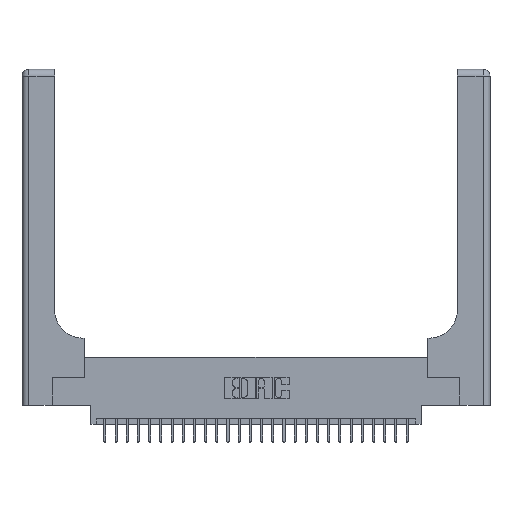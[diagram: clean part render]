
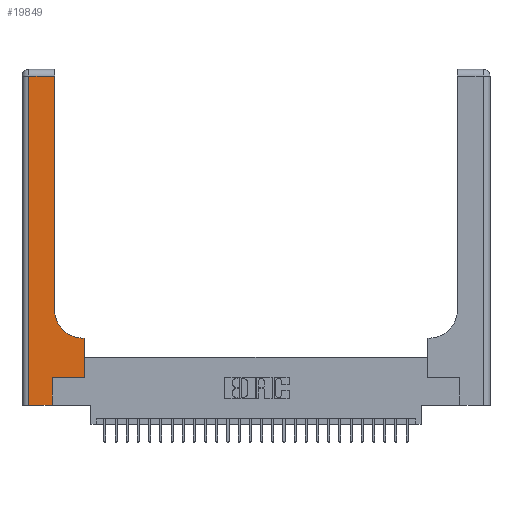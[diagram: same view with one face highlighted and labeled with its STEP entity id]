
A CAD part, top view. The second image highlights one B-rep face of the part: STEP entity #19849.
In plain terms, the highlighted planar face has unit normal (0, 0, 1).
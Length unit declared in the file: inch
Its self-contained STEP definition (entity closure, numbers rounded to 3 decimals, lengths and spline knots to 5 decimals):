
#695 = ORIENTED_EDGE ( 'NONE', *, *, #17279, .T. ) ;
#705 = CARTESIAN_POINT ( 'NONE',  ( 0.269, 0., 0.37 ) ) ;
#976 = VERTEX_POINT ( 'NONE', #12389 ) ;
#1508 = VERTEX_POINT ( 'NONE', #21222 ) ;
#1561 = CARTESIAN_POINT ( 'NONE',  ( 0.269, 0.25, 0.37 ) ) ;
#1582 = CARTESIAN_POINT ( 'NONE',  ( 0.06, 2.94, 0.37 ) ) ;
#2158 = CARTESIAN_POINT ( 'NONE',  ( 0.06, 3., 0.37 ) ) ;
#2803 = FACE_OUTER_BOUND ( 'NONE', #26682, .T. ) ;
#2903 = VERTEX_POINT ( 'NONE', #705 ) ;
#3020 = DIRECTION ( 'NONE',  ( 0., 1., 0. ) ) ;
#3133 = CARTESIAN_POINT ( 'NONE',  ( 0.5415, 0.85, 0.37 ) ) ;
#3199 = LINE ( 'NONE', #19213, #16576 ) ;
#3409 = VECTOR ( 'NONE', #8537, 39.37008 ) ;
#3973 = CARTESIAN_POINT ( 'NONE',  ( 0.2915, 0.85, 0.37 ) ) ;
#4319 = EDGE_CURVE ( 'NONE', #24713, #976, #20401, .T. ) ;
#5251 = VECTOR ( 'NONE', #23430, 39.37008 ) ;
#5928 = ORIENTED_EDGE ( 'NONE', *, *, #14879, .T. ) ;
#6077 = EDGE_CURVE ( 'NONE', #976, #27820, #9397, .T. ) ;
#6463 = CARTESIAN_POINT ( 'NONE',  ( 0., 2.94, 0.37 ) ) ;
#7162 = LINE ( 'NONE', #2158, #20213 ) ;
#7233 = VERTEX_POINT ( 'NONE', #18867 ) ;
#7284 = EDGE_CURVE ( 'NONE', #23984, #1508, #7162, .T. ) ;
#7417 = ORIENTED_EDGE ( 'NONE', *, *, #4319, .T. ) ;
#7922 = EDGE_CURVE ( 'NONE', #27820, #7233, #22665, .T. ) ;
#8462 = AXIS2_PLACEMENT_3D ( 'NONE', #21516, #21420, #23816 ) ;
#8537 = DIRECTION ( 'NONE',  ( -1., 0., 0. ) ) ;
#8786 = DIRECTION ( 'NONE',  ( 0., -1., 0. ) ) ;
#9397 = LINE ( 'NONE', #21067, #14976 ) ;
#9535 = DIRECTION ( 'NONE',  ( 0., 1., 0. ) ) ;
#9576 = EDGE_CURVE ( 'NONE', #7233, #25242, #14083, .T. ) ;
#10466 = LINE ( 'NONE', #11549, #18860 ) ;
#10590 = ORIENTED_EDGE ( 'NONE', *, *, #9576, .T. ) ;
#10990 = VECTOR ( 'NONE', #9535, 39.37008 ) ;
#11549 = CARTESIAN_POINT ( 'NONE',  ( 0., 0., 0.37 ) ) ;
#12389 = CARTESIAN_POINT ( 'NONE',  ( 0.5585, 0.25, 0.37 ) ) ;
#13923 = LINE ( 'NONE', #6463, #3409 ) ;
#14083 = CIRCLE ( 'NONE', #21953, 0.25 ) ;
#14301 = EDGE_CURVE ( 'NONE', #24457, #23984, #13923, .T. ) ;
#14713 = CARTESIAN_POINT ( 'NONE',  ( 0.2915, 3., 0.37 ) ) ;
#14879 = EDGE_CURVE ( 'NONE', #1508, #2903, #10466, .T. ) ;
#14976 = VECTOR ( 'NONE', #3020, 39.37008 ) ;
#15529 = CARTESIAN_POINT ( 'NONE',  ( 0.5585, 0.6, 0.37 ) ) ;
#16576 = VECTOR ( 'NONE', #24003, 39.37008 ) ;
#17279 = EDGE_CURVE ( 'NONE', #25242, #24457, #27245, .T. ) ;
#18101 = VECTOR ( 'NONE', #26545, 39.37008 ) ;
#18860 = VECTOR ( 'NONE', #28061, 39.37008 ) ;
#18867 = CARTESIAN_POINT ( 'NONE',  ( 0.5415, 0.6, 0.37 ) ) ;
#19060 = ORIENTED_EDGE ( 'NONE', *, *, #7922, .T. ) ;
#19213 = CARTESIAN_POINT ( 'NONE',  ( 0.269, 0., 0.37 ) ) ;
#19849 = ADVANCED_FACE ( 'NONE', ( #2803 ), #28256, .F. ) ;
#20213 = VECTOR ( 'NONE', #8786, 39.37008 ) ;
#20401 = LINE ( 'NONE', #21445, #5251 ) ;
#20995 = DIRECTION ( 'NONE',  ( 0., 0., -1. ) ) ;
#21067 = CARTESIAN_POINT ( 'NONE',  ( 0.5585, 0.25, 0.37 ) ) ;
#21222 = CARTESIAN_POINT ( 'NONE',  ( 0.06, 0., 0.37 ) ) ;
#21420 = DIRECTION ( 'NONE',  ( 0., 0., -1. ) ) ;
#21430 = ORIENTED_EDGE ( 'NONE', *, *, #25839, .T. ) ;
#21445 = CARTESIAN_POINT ( 'NONE',  ( 0.269, 0.25, 0.37 ) ) ;
#21516 = CARTESIAN_POINT ( 'NONE',  ( 0., 3., 0.37 ) ) ;
#21953 = AXIS2_PLACEMENT_3D ( 'NONE', #3133, #20995, #25650 ) ;
#21979 = ORIENTED_EDGE ( 'NONE', *, *, #6077, .T. ) ;
#22665 = LINE ( 'NONE', #24667, #18101 ) ;
#23430 = DIRECTION ( 'NONE',  ( 1., 0., 0. ) ) ;
#23816 = DIRECTION ( 'NONE',  ( -1., 0., 0. ) ) ;
#23984 = VERTEX_POINT ( 'NONE', #1582 ) ;
#24003 = DIRECTION ( 'NONE',  ( 0., 1., 0. ) ) ;
#24457 = VERTEX_POINT ( 'NONE', #28130 ) ;
#24667 = CARTESIAN_POINT ( 'NONE',  ( 0.2915, 0.6, 0.37 ) ) ;
#24713 = VERTEX_POINT ( 'NONE', #1561 ) ;
#24883 = ORIENTED_EDGE ( 'NONE', *, *, #14301, .T. ) ;
#25242 = VERTEX_POINT ( 'NONE', #3973 ) ;
#25650 = DIRECTION ( 'NONE',  ( 1., 0., 0. ) ) ;
#25839 = EDGE_CURVE ( 'NONE', #2903, #24713, #3199, .T. ) ;
#25946 = ORIENTED_EDGE ( 'NONE', *, *, #7284, .T. ) ;
#26545 = DIRECTION ( 'NONE',  ( -1., 0., 0. ) ) ;
#26682 = EDGE_LOOP ( 'NONE', ( #695, #24883, #25946, #5928, #21430, #7417, #21979, #19060, #10590 ) ) ;
#27245 = LINE ( 'NONE', #14713, #10990 ) ;
#27820 = VERTEX_POINT ( 'NONE', #15529 ) ;
#28061 = DIRECTION ( 'NONE',  ( 1., 0., 0. ) ) ;
#28130 = CARTESIAN_POINT ( 'NONE',  ( 0.2915, 2.94, 0.37 ) ) ;
#28256 = PLANE ( 'NONE',  #8462 ) ;
